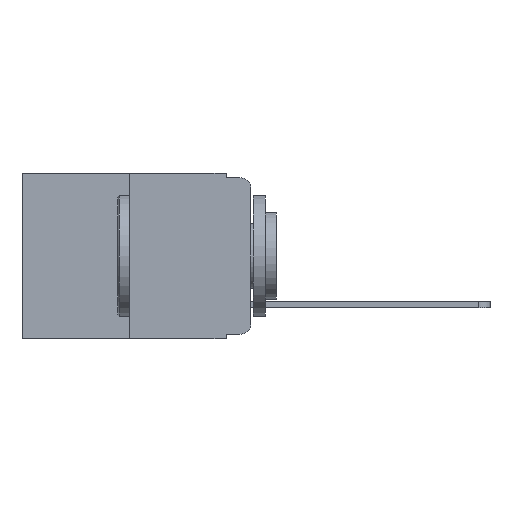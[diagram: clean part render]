
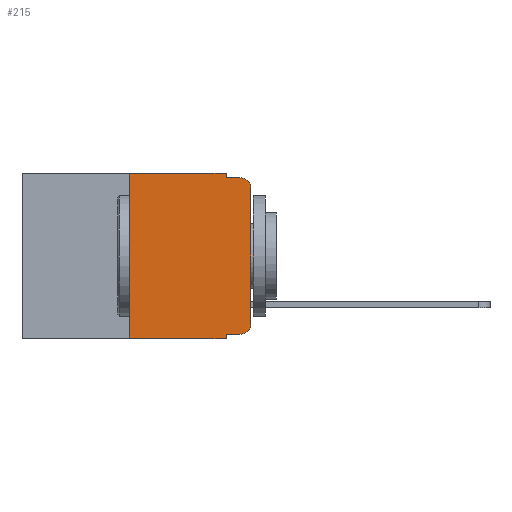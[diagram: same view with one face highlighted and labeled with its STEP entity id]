
A CAD part, left-side view. The second image highlights one B-rep face of the part: STEP entity #215.
In plain terms, the highlighted planar face has unit normal (-1, 0, 0).
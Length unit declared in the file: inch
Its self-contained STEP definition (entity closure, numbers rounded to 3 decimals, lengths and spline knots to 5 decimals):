
#172 = CARTESIAN_POINT ( 'NONE',  ( 0., 0.02, -0.01 ) ) ;
#215 = ADVANCED_FACE ( 'NONE', ( #17898 ), #12825, .F. ) ;
#403 = DIRECTION ( 'NONE',  ( 0., 0., 1. ) ) ;
#532 = VERTEX_POINT ( 'NONE', #1028 ) ;
#993 = CIRCLE ( 'NONE', #8058, 0.02 ) ;
#1028 = CARTESIAN_POINT ( 'NONE',  ( 0., 0.25, -0.343 ) ) ;
#1528 = ORIENTED_EDGE ( 'NONE', *, *, #3818, .T. ) ;
#1975 = ORIENTED_EDGE ( 'NONE', *, *, #3443, .T. ) ;
#2332 = ORIENTED_EDGE ( 'NONE', *, *, #3941, .T. ) ;
#2538 = CARTESIAN_POINT ( 'NONE',  ( 0., 0.051, -0.333 ) ) ;
#2658 = CIRCLE ( 'NONE', #17223, 0.02 ) ;
#2834 = DIRECTION ( 'NONE',  ( 0., -1., 0. ) ) ;
#2886 = CARTESIAN_POINT ( 'NONE',  ( 0., 0.051, 0. ) ) ;
#2951 = EDGE_CURVE ( 'NONE', #10656, #5989, #11605, .T. ) ;
#3102 = VERTEX_POINT ( 'NONE', #5439 ) ;
#3292 = VECTOR ( 'NONE', #8449, 39.37008 ) ;
#3443 = EDGE_CURVE ( 'NONE', #532, #17562, #21112, .T. ) ;
#3695 = CARTESIAN_POINT ( 'NONE',  ( 0., 0.051, -0.333 ) ) ;
#3761 = VERTEX_POINT ( 'NONE', #5980 ) ;
#3818 = EDGE_CURVE ( 'NONE', #22773, #3761, #6972, .T. ) ;
#3823 = EDGE_CURVE ( 'NONE', #3761, #15268, #993, .T. ) ;
#3860 = EDGE_CURVE ( 'NONE', #16936, #15268, #14626, .T. ) ;
#3884 = LINE ( 'NONE', #2538, #7886 ) ;
#3902 = EDGE_CURVE ( 'NONE', #5989, #16936, #18548, .T. ) ;
#3910 = EDGE_CURVE ( 'NONE', #532, #10656, #9598, .T. ) ;
#3917 = DIRECTION ( 'NONE',  ( 0., -1., 0. ) ) ;
#3933 = EDGE_CURVE ( 'NONE', #20432, #17562, #13044, .T. ) ;
#3941 = EDGE_CURVE ( 'NONE', #20432, #3102, #3884, .T. ) ;
#3966 = EDGE_CURVE ( 'NONE', #3102, #22773, #2658, .T. ) ;
#4665 = CARTESIAN_POINT ( 'NONE',  ( 0., 0.473, 0. ) ) ;
#5050 = DIRECTION ( 'NONE',  ( 1., 0., 0. ) ) ;
#5439 = CARTESIAN_POINT ( 'NONE',  ( 0., 0.02, -0.333 ) ) ;
#5515 = DIRECTION ( 'NONE',  ( 0., 0., -1. ) ) ;
#5980 = CARTESIAN_POINT ( 'NONE',  ( 0., 0., -0.03 ) ) ;
#5989 = VERTEX_POINT ( 'NONE', #2886 ) ;
#6227 = CARTESIAN_POINT ( 'NONE',  ( 0., 0.02, -0.03 ) ) ;
#6347 = VECTOR ( 'NONE', #9938, 39.37008 ) ;
#6406 = CARTESIAN_POINT ( 'NONE',  ( 0., 0.051, 0. ) ) ;
#6615 = CARTESIAN_POINT ( 'NONE',  ( 0., 0.051, -0.01 ) ) ;
#6780 = CARTESIAN_POINT ( 'NONE',  ( 0., 0.473, -0.343 ) ) ;
#6783 = VECTOR ( 'NONE', #3917, 39.37008 ) ;
#6972 = LINE ( 'NONE', #8128, #6347 ) ;
#7096 = CARTESIAN_POINT ( 'NONE',  ( 0., 0., -0.313 ) ) ;
#7886 = VECTOR ( 'NONE', #17019, 39.37008 ) ;
#8058 = AXIS2_PLACEMENT_3D ( 'NONE', #6227, #18379, #8224 ) ;
#8128 = CARTESIAN_POINT ( 'NONE',  ( 0., 0., 0. ) ) ;
#8224 = DIRECTION ( 'NONE',  ( 0., 0., -1. ) ) ;
#8449 = DIRECTION ( 'NONE',  ( 0., 0., -1. ) ) ;
#8597 = DIRECTION ( 'NONE',  ( -1., 0., 0. ) ) ;
#9078 = AXIS2_PLACEMENT_3D ( 'NONE', #12840, #5050, #5515 ) ;
#9598 = LINE ( 'NONE', #21787, #21847 ) ;
#9938 = DIRECTION ( 'NONE',  ( 0., 0., 1. ) ) ;
#10234 = CARTESIAN_POINT ( 'NONE',  ( 0., 0.051, 0. ) ) ;
#10656 = VERTEX_POINT ( 'NONE', #16989 ) ;
#11605 = LINE ( 'NONE', #4665, #6783 ) ;
#12303 = VECTOR ( 'NONE', #2834, 39.37008 ) ;
#12779 = ORIENTED_EDGE ( 'NONE', *, *, #3966, .T. ) ;
#12825 = PLANE ( 'NONE',  #9078 ) ;
#12840 = CARTESIAN_POINT ( 'NONE',  ( 0., 0.473, 0. ) ) ;
#13044 = LINE ( 'NONE', #10234, #3292 ) ;
#13221 = ORIENTED_EDGE ( 'NONE', *, *, #3823, .T. ) ;
#13512 = ORIENTED_EDGE ( 'NONE', *, *, #3860, .F. ) ;
#13561 = ORIENTED_EDGE ( 'NONE', *, *, #3933, .F. ) ;
#13817 = ORIENTED_EDGE ( 'NONE', *, *, #2951, .F. ) ;
#14626 = LINE ( 'NONE', #18443, #22883 ) ;
#15268 = VERTEX_POINT ( 'NONE', #172 ) ;
#15408 = ORIENTED_EDGE ( 'NONE', *, *, #3910, .F. ) ;
#16936 = VERTEX_POINT ( 'NONE', #6615 ) ;
#16989 = CARTESIAN_POINT ( 'NONE',  ( 0., 0.25, 0. ) ) ;
#17019 = DIRECTION ( 'NONE',  ( 0., -1., 0. ) ) ;
#17223 = AXIS2_PLACEMENT_3D ( 'NONE', #18730, #8597, #20366 ) ;
#17562 = VERTEX_POINT ( 'NONE', #21600 ) ;
#17898 = FACE_OUTER_BOUND ( 'NONE', #20523, .T. ) ;
#18015 = VECTOR ( 'NONE', #18525, 39.37008 ) ;
#18379 = DIRECTION ( 'NONE',  ( -1., 0., 0. ) ) ;
#18443 = CARTESIAN_POINT ( 'NONE',  ( 0., 0.051, -0.01 ) ) ;
#18525 = DIRECTION ( 'NONE',  ( 0., 0., -1. ) ) ;
#18548 = LINE ( 'NONE', #6406, #18015 ) ;
#18730 = CARTESIAN_POINT ( 'NONE',  ( 0., 0.02, -0.313 ) ) ;
#20088 = DIRECTION ( 'NONE',  ( 0., -1., 0. ) ) ;
#20366 = DIRECTION ( 'NONE',  ( 0., 0., -1. ) ) ;
#20432 = VERTEX_POINT ( 'NONE', #3695 ) ;
#20523 = EDGE_LOOP ( 'NONE', ( #1528, #13221, #13512, #21308, #13817, #15408, #1975, #13561, #2332, #12779 ) ) ;
#21112 = LINE ( 'NONE', #6780, #12303 ) ;
#21308 = ORIENTED_EDGE ( 'NONE', *, *, #3902, .F. ) ;
#21600 = CARTESIAN_POINT ( 'NONE',  ( 0., 0.051, -0.343 ) ) ;
#21787 = CARTESIAN_POINT ( 'NONE',  ( 0., 0.25, 0. ) ) ;
#21847 = VECTOR ( 'NONE', #403, 39.37008 ) ;
#22773 = VERTEX_POINT ( 'NONE', #7096 ) ;
#22883 = VECTOR ( 'NONE', #20088, 39.37008 ) ;
